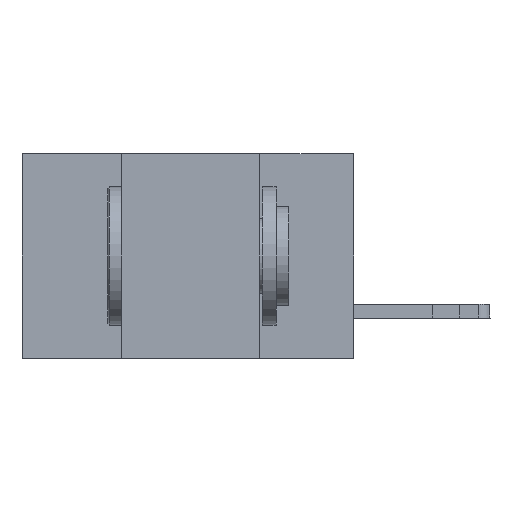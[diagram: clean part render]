
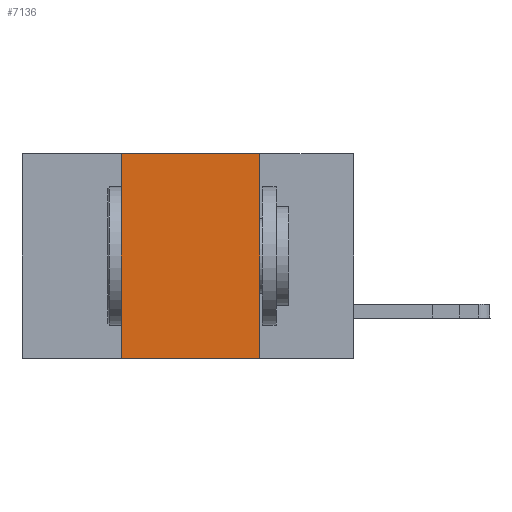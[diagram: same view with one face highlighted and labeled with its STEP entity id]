
A CAD part, left-side view. The second image highlights one B-rep face of the part: STEP entity #7136.
In plain terms, the highlighted planar face has unit normal (-1, 0, 0).
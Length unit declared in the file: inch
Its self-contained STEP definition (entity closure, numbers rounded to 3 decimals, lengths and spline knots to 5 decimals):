
#420 = DIRECTION ( 'NONE',  ( 0., 0., -1. ) ) ;
#732 = CARTESIAN_POINT ( 'NONE',  ( 0., 0.42, -0.37 ) ) ;
#783 = VERTEX_POINT ( 'NONE', #13294 ) ;
#1737 = CARTESIAN_POINT ( 'NONE',  ( 0., 0.6, 0. ) ) ;
#1863 = VECTOR ( 'NONE', #420, 39.37008 ) ;
#3024 = ORIENTED_EDGE ( 'NONE', *, *, #10837, .F. ) ;
#3279 = EDGE_CURVE ( 'NONE', #24998, #4514, #8261, .T. ) ;
#4514 = VERTEX_POINT ( 'NONE', #18479 ) ;
#5457 = ORIENTED_EDGE ( 'NONE', *, *, #13067, .F. ) ;
#7136 = ADVANCED_FACE ( 'NONE', ( #17624 ), #8377, .F. ) ;
#8194 = LINE ( 'NONE', #25769, #1863 ) ;
#8261 = LINE ( 'NONE', #16118, #18872 ) ;
#8377 = PLANE ( 'NONE',  #10153 ) ;
#10153 = AXIS2_PLACEMENT_3D ( 'NONE', #12663, #27285, #14795 ) ;
#10837 = EDGE_CURVE ( 'NONE', #16639, #4514, #8194, .T. ) ;
#10910 = LINE ( 'NONE', #1737, #26982 ) ;
#12663 = CARTESIAN_POINT ( 'NONE',  ( 0., 0.6, 0. ) ) ;
#13067 = EDGE_CURVE ( 'NONE', #24998, #783, #24204, .T. ) ;
#13294 = CARTESIAN_POINT ( 'NONE',  ( 0., 0.42, 0. ) ) ;
#14795 = DIRECTION ( 'NONE',  ( 0., 0., -1. ) ) ;
#16118 = CARTESIAN_POINT ( 'NONE',  ( 0., 0.6, -0.37 ) ) ;
#16212 = DIRECTION ( 'NONE',  ( 0., -1., 0. ) ) ;
#16215 = ORIENTED_EDGE ( 'NONE', *, *, #3279, .T. ) ;
#16639 = VERTEX_POINT ( 'NONE', #26988 ) ;
#17624 = FACE_OUTER_BOUND ( 'NONE', #25822, .T. ) ;
#18479 = CARTESIAN_POINT ( 'NONE',  ( 0., 0.17, -0.37 ) ) ;
#18660 = VECTOR ( 'NONE', #27014, 39.37008 ) ;
#18667 = CARTESIAN_POINT ( 'NONE',  ( 0., 0.42, 0. ) ) ;
#18872 = VECTOR ( 'NONE', #16212, 39.37008 ) ;
#20345 = ORIENTED_EDGE ( 'NONE', *, *, #24039, .F. ) ;
#24039 = EDGE_CURVE ( 'NONE', #783, #16639, #10910, .T. ) ;
#24204 = LINE ( 'NONE', #18667, #18660 ) ;
#24998 = VERTEX_POINT ( 'NONE', #732 ) ;
#25769 = CARTESIAN_POINT ( 'NONE',  ( 0., 0.17, 0. ) ) ;
#25822 = EDGE_LOOP ( 'NONE', ( #3024, #20345, #5457, #16215 ) ) ;
#26982 = VECTOR ( 'NONE', #27092, 39.37008 ) ;
#26988 = CARTESIAN_POINT ( 'NONE',  ( 0., 0.17, 0. ) ) ;
#27014 = DIRECTION ( 'NONE',  ( 0., 0., 1. ) ) ;
#27092 = DIRECTION ( 'NONE',  ( 0., -1., 0. ) ) ;
#27285 = DIRECTION ( 'NONE',  ( 1., 0., 0. ) ) ;
